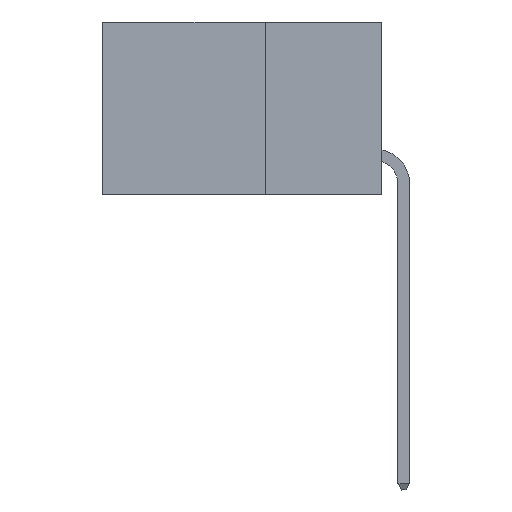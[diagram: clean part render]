
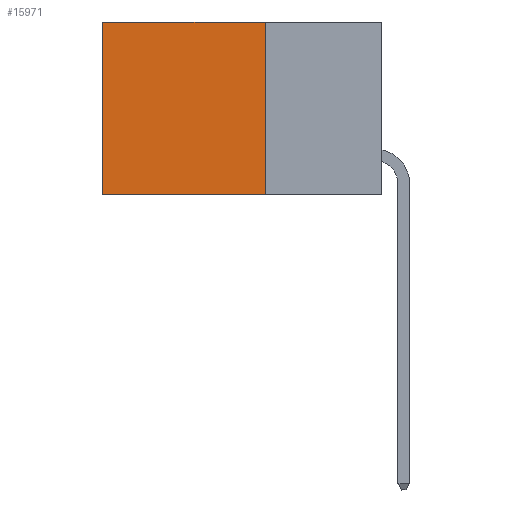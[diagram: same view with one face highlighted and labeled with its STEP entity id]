
A CAD part, left-side view. The second image highlights one B-rep face of the part: STEP entity #15971.
In plain terms, the highlighted planar face has unit normal (-1, 0, 0).
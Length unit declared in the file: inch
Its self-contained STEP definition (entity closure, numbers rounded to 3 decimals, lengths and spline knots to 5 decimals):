
#726 = VECTOR ( 'NONE', #28680, 39.37008 ) ;
#1257 = VECTOR ( 'NONE', #37602, 39.37008 ) ;
#3343 = PLANE ( 'NONE',  #37474 ) ;
#3748 = DIRECTION ( 'NONE',  ( 1., 0., 0. ) ) ;
#4041 = CARTESIAN_POINT ( 'NONE',  ( 0.2875, 0.25, 0. ) ) ;
#4635 = LINE ( 'NONE', #23084, #20998 ) ;
#5145 = VERTEX_POINT ( 'NONE', #29869 ) ;
#5605 = CARTESIAN_POINT ( 'NONE',  ( 0.2875, 0.25, 0. ) ) ;
#8221 = VECTOR ( 'NONE', #18853, 39.37008 ) ;
#9155 = EDGE_LOOP ( 'NONE', ( #15465, #11248, #25728, #18215 ) ) ;
#9958 = DIRECTION ( 'NONE',  ( 0., 0., -1. ) ) ;
#10692 = VERTEX_POINT ( 'NONE', #24404 ) ;
#11248 = ORIENTED_EDGE ( 'NONE', *, *, #41211, .F. ) ;
#12142 = EDGE_CURVE ( 'NONE', #10692, #19922, #4635, .T. ) ;
#15465 = ORIENTED_EDGE ( 'NONE', *, *, #12142, .T. ) ;
#15971 = ADVANCED_FACE ( 'NONE', ( #25472 ), #3343, .F. ) ;
#18215 = ORIENTED_EDGE ( 'NONE', *, *, #28229, .T. ) ;
#18853 = DIRECTION ( 'NONE',  ( 0., 0., -1. ) ) ;
#19922 = VERTEX_POINT ( 'NONE', #19961 ) ;
#19961 = CARTESIAN_POINT ( 'NONE',  ( 0.2875, 0.6, -0.37 ) ) ;
#20019 = CARTESIAN_POINT ( 'NONE',  ( 0.2875, 0.25, 0. ) ) ;
#20998 = VECTOR ( 'NONE', #9958, 39.37008 ) ;
#21223 = LINE ( 'NONE', #41730, #726 ) ;
#23084 = CARTESIAN_POINT ( 'NONE',  ( 0.2875, 0.6, 0. ) ) ;
#23800 = VERTEX_POINT ( 'NONE', #4041 ) ;
#24404 = CARTESIAN_POINT ( 'NONE',  ( 0.2875, 0.6, 0. ) ) ;
#24457 = EDGE_CURVE ( 'NONE', #23800, #5145, #30589, .T. ) ;
#25472 = FACE_OUTER_BOUND ( 'NONE', #9155, .T. ) ;
#25728 = ORIENTED_EDGE ( 'NONE', *, *, #24457, .F. ) ;
#26333 = DIRECTION ( 'NONE',  ( 0., 0., -1. ) ) ;
#27853 = LINE ( 'NONE', #31220, #1257 ) ;
#28229 = EDGE_CURVE ( 'NONE', #23800, #10692, #21223, .T. ) ;
#28680 = DIRECTION ( 'NONE',  ( 0., 1., 0. ) ) ;
#29869 = CARTESIAN_POINT ( 'NONE',  ( 0.2875, 0.25, -0.37 ) ) ;
#30589 = LINE ( 'NONE', #5605, #8221 ) ;
#31220 = CARTESIAN_POINT ( 'NONE',  ( 0.2875, 0.25, -0.37 ) ) ;
#37474 = AXIS2_PLACEMENT_3D ( 'NONE', #20019, #3748, #26333 ) ;
#37602 = DIRECTION ( 'NONE',  ( 0., 1., 0. ) ) ;
#41211 = EDGE_CURVE ( 'NONE', #5145, #19922, #27853, .T. ) ;
#41730 = CARTESIAN_POINT ( 'NONE',  ( 0.2875, 0.25, 0. ) ) ;
